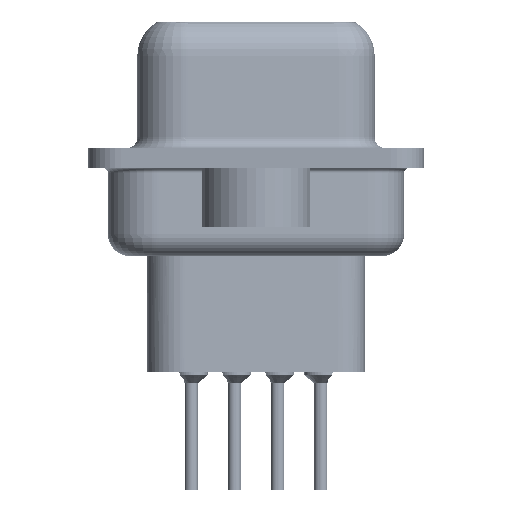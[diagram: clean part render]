
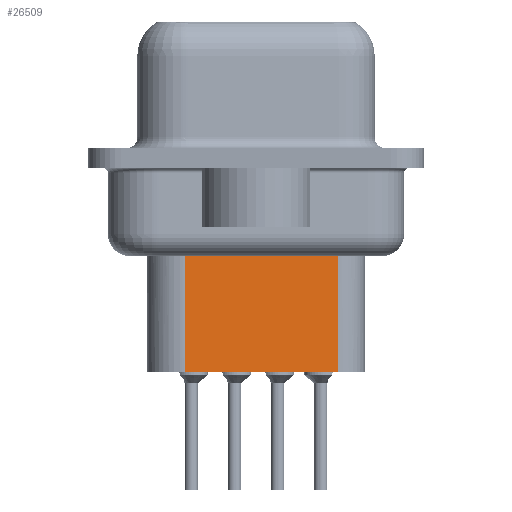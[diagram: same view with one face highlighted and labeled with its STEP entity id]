
A CAD part, left-side view. The second image highlights one B-rep face of the part: STEP entity #26509.
In plain terms, the highlighted planar face has unit normal (-0.985, -0.174, 0).
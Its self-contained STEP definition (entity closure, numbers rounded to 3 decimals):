
#1583 = EDGE_CURVE ( 'NONE', #50307, #38807, #37297, .T. ) ;
#2751 = CARTESIAN_POINT ( 'NONE',  ( 4.453, 4.209, -3.975 ) ) ;
#3055 = DIRECTION ( 'NONE',  ( -0.985, -0.174, 0. ) ) ;
#4870 = CARTESIAN_POINT ( 'NONE',  ( 4.624, 3.24, -3.1 ) ) ;
#5069 = EDGE_CURVE ( 'NONE', #50307, #53960, #34795, .T. ) ;
#5677 = VECTOR ( 'NONE', #10633, 1000. ) ;
#5731 = DIRECTION ( 'NONE',  ( 0., 0., -1. ) ) ;
#7434 = DIRECTION ( 'NONE',  ( 0.174, -0.985, 0. ) ) ;
#7720 = FACE_OUTER_BOUND ( 'NONE', #48432, .T. ) ;
#10633 = DIRECTION ( 'NONE',  ( -0.174, 0.985, 0. ) ) ;
#12505 = CARTESIAN_POINT ( 'NONE',  ( 4.624, 3.24, -9.85 ) ) ;
#19088 = CARTESIAN_POINT ( 'NONE',  ( 5.858, -3.76, -3.975 ) ) ;
#19586 = VECTOR ( 'NONE', #57001, 1000. ) ;
#21418 = PLANE ( 'NONE',  #29980 ) ;
#22065 = CARTESIAN_POINT ( 'NONE',  ( 5.858, -3.76, -9.85 ) ) ;
#23347 = ORIENTED_EDGE ( 'NONE', *, *, #49913, .T. ) ;
#25671 = ORIENTED_EDGE ( 'NONE', *, *, #42536, .F. ) ;
#26509 = ADVANCED_FACE ( 'NONE', ( #7720 ), #21418, .T. ) ;
#26621 = VECTOR ( 'NONE', #51498, 1000. ) ;
#29980 = AXIS2_PLACEMENT_3D ( 'NONE', #38388, #3055, #7434 ) ;
#33374 = CARTESIAN_POINT ( 'NONE',  ( 4.624, 3.24, -9.85 ) ) ;
#34065 = VECTOR ( 'NONE', #5731, 1000. ) ;
#34437 = ORIENTED_EDGE ( 'NONE', *, *, #5069, .F. ) ;
#34795 = LINE ( 'NONE', #48535, #19586 ) ;
#35157 = CARTESIAN_POINT ( 'NONE',  ( 4.624, 3.24, -3.975 ) ) ;
#36396 = LINE ( 'NONE', #4870, #34065 ) ;
#37297 = LINE ( 'NONE', #2751, #26621 ) ;
#38388 = CARTESIAN_POINT ( 'NONE',  ( 4.624, 3.24, -3.1 ) ) ;
#38807 = VERTEX_POINT ( 'NONE', #35157 ) ;
#39163 = ORIENTED_EDGE ( 'NONE', *, *, #1583, .T. ) ;
#42536 = EDGE_CURVE ( 'NONE', #53960, #48630, #46539, .T. ) ;
#46539 = LINE ( 'NONE', #33374, #5677 ) ;
#48432 = EDGE_LOOP ( 'NONE', ( #34437, #39163, #23347, #25671 ) ) ;
#48535 = CARTESIAN_POINT ( 'NONE',  ( 5.858, -3.76, -3.1 ) ) ;
#48630 = VERTEX_POINT ( 'NONE', #12505 ) ;
#49913 = EDGE_CURVE ( 'NONE', #38807, #48630, #36396, .T. ) ;
#50307 = VERTEX_POINT ( 'NONE', #19088 ) ;
#51498 = DIRECTION ( 'NONE',  ( -0.174, 0.985, 0. ) ) ;
#53960 = VERTEX_POINT ( 'NONE', #22065 ) ;
#57001 = DIRECTION ( 'NONE',  ( 0., 0., -1. ) ) ;
